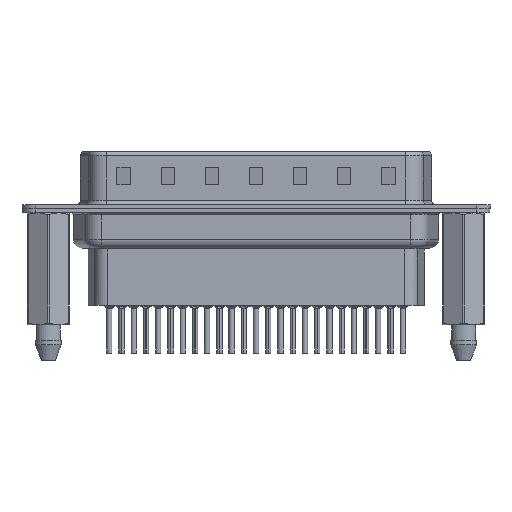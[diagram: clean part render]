
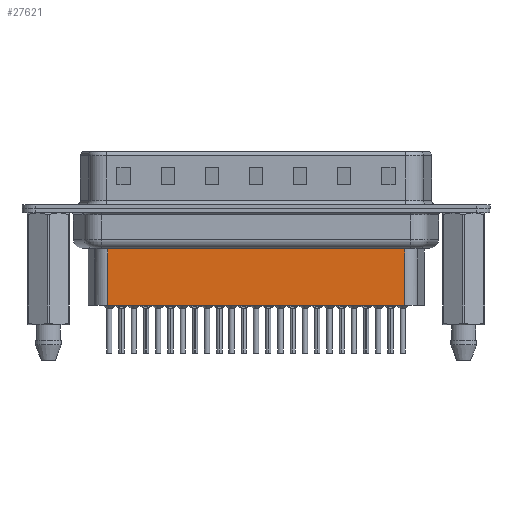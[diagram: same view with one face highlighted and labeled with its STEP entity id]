
A CAD part, front view. The second image highlights one B-rep face of the part: STEP entity #27621.
In plain terms, the highlighted planar face has unit normal (0, -1, 0).
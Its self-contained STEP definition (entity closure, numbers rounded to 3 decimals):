
#151 = DIRECTION ( 'NONE',  ( 0., 0., -1. ) ) ;
#342 = VECTOR ( 'NONE', #20303, 1000. ) ;
#723 = CARTESIAN_POINT ( 'NONE',  ( 6.706, -3.5, -3.1 ) ) ;
#1871 = VECTOR ( 'NONE', #27284, 1000. ) ;
#4932 = DIRECTION ( 'NONE',  ( -1., 0., 0. ) ) ;
#5185 = ORIENTED_EDGE ( 'NONE', *, *, #16956, .F. ) ;
#5756 = VERTEX_POINT ( 'NONE', #15493 ) ;
#6222 = CARTESIAN_POINT ( 'NONE',  ( 6.706, -3.5, -10.95 ) ) ;
#6842 = VERTEX_POINT ( 'NONE', #16842 ) ;
#7988 = DIRECTION ( 'NONE',  ( 0., -1., 0. ) ) ;
#8009 = ORIENTED_EDGE ( 'NONE', *, *, #13356, .T. ) ;
#9025 = LINE ( 'NONE', #723, #19586 ) ;
#9079 = VECTOR ( 'NONE', #4932, 1000. ) ;
#9344 = CARTESIAN_POINT ( 'NONE',  ( 6.459, -3.5, -4.097 ) ) ;
#11550 = CARTESIAN_POINT ( 'NONE',  ( 6.706, -3.5, -10.95 ) ) ;
#11796 = LINE ( 'NONE', #11550, #9079 ) ;
#12371 = CARTESIAN_POINT ( 'NONE',  ( 6.706, -3.5, -3.1 ) ) ;
#13356 = EDGE_CURVE ( 'NONE', #5756, #21219, #9025, .T. ) ;
#13855 = CARTESIAN_POINT ( 'NONE',  ( 40.344, -3.5, -10.95 ) ) ;
#14162 = ORIENTED_EDGE ( 'NONE', *, *, #16787, .F. ) ;
#14787 = AXIS2_PLACEMENT_3D ( 'NONE', #12371, #7988, #16718 ) ;
#15493 = CARTESIAN_POINT ( 'NONE',  ( 6.706, -3.5, -4.097 ) ) ;
#15804 = LINE ( 'NONE', #9344, #342 ) ;
#16445 = FACE_OUTER_BOUND ( 'NONE', #20875, .T. ) ;
#16718 = DIRECTION ( 'NONE',  ( 1., 0., 0. ) ) ;
#16787 = EDGE_CURVE ( 'NONE', #23219, #21219, #11796, .T. ) ;
#16842 = CARTESIAN_POINT ( 'NONE',  ( 40.344, -3.5, -4.097 ) ) ;
#16956 = EDGE_CURVE ( 'NONE', #6842, #23219, #18704, .T. ) ;
#18704 = LINE ( 'NONE', #23060, #1871 ) ;
#19586 = VECTOR ( 'NONE', #151, 1000. ) ;
#20303 = DIRECTION ( 'NONE',  ( -1., 0., 0. ) ) ;
#20875 = EDGE_LOOP ( 'NONE', ( #5185, #22115, #8009, #14162 ) ) ;
#21219 = VERTEX_POINT ( 'NONE', #6222 ) ;
#22115 = ORIENTED_EDGE ( 'NONE', *, *, #25191, .T. ) ;
#23060 = CARTESIAN_POINT ( 'NONE',  ( 40.344, -3.5, -3.1 ) ) ;
#23219 = VERTEX_POINT ( 'NONE', #13855 ) ;
#25191 = EDGE_CURVE ( 'NONE', #6842, #5756, #15804, .T. ) ;
#27284 = DIRECTION ( 'NONE',  ( 0., 0., -1. ) ) ;
#27410 = PLANE ( 'NONE',  #14787 ) ;
#27621 = ADVANCED_FACE ( 'NONE', ( #16445 ), #27410, .T. ) ;
